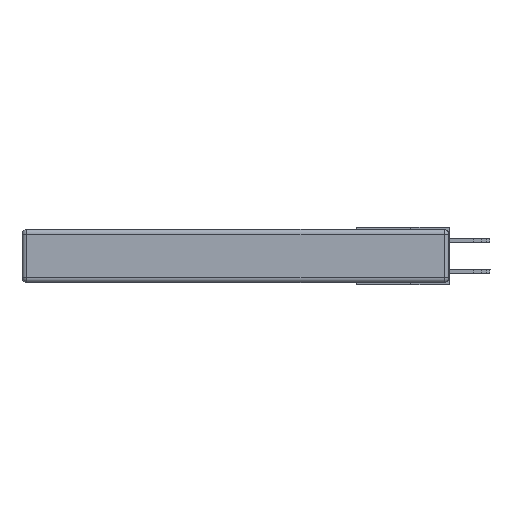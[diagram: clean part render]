
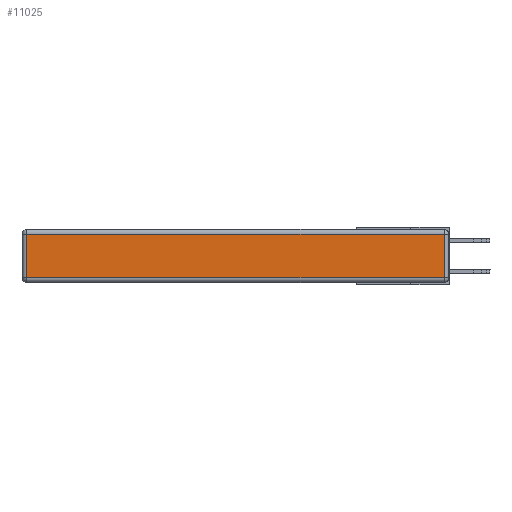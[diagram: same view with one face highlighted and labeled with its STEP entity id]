
A CAD part, left-side view. The second image highlights one B-rep face of the part: STEP entity #11025.
In plain terms, the highlighted planar face has unit normal (-1, 0, 0).
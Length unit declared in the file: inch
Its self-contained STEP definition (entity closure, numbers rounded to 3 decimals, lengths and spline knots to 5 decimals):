
#323 = DIRECTION ( 'NONE',  ( 0., -1., 0. ) ) ;
#461 = AXIS2_PLACEMENT_3D ( 'NONE', #13954, #5909, #7148 ) ;
#526 = VECTOR ( 'NONE', #9962, 39.37008 ) ;
#1801 = LINE ( 'NONE', #3574, #526 ) ;
#1982 = CARTESIAN_POINT ( 'NONE',  ( 0., 0.03, -0.313 ) ) ;
#2169 = DIRECTION ( 'NONE',  ( 0., 1., 0. ) ) ;
#2278 = VERTEX_POINT ( 'NONE', #8312 ) ;
#3091 = EDGE_CURVE ( 'NONE', #2278, #4308, #16827, .T. ) ;
#3574 = CARTESIAN_POINT ( 'NONE',  ( 0., 0.03, -0.343 ) ) ;
#4308 = VERTEX_POINT ( 'NONE', #16185 ) ;
#4618 = DIRECTION ( 'NONE',  ( 0., 0., -1. ) ) ;
#4994 = VECTOR ( 'NONE', #2169, 39.37008 ) ;
#5675 = CARTESIAN_POINT ( 'NONE',  ( 0., 0., -0.313 ) ) ;
#5909 = DIRECTION ( 'NONE',  ( -1., 0., 0. ) ) ;
#6187 = CARTESIAN_POINT ( 'NONE',  ( 0., 2.75, -0.03 ) ) ;
#6301 = CARTESIAN_POINT ( 'NONE',  ( 0., 0.03, -0.03 ) ) ;
#6712 = VECTOR ( 'NONE', #4618, 39.37008 ) ;
#7148 = DIRECTION ( 'NONE',  ( 0., 0., 1. ) ) ;
#7435 = CARTESIAN_POINT ( 'NONE',  ( 0., 2.72, -0.343 ) ) ;
#8312 = CARTESIAN_POINT ( 'NONE',  ( 0., 2.72, -0.03 ) ) ;
#9962 = DIRECTION ( 'NONE',  ( 0., 0., 1. ) ) ;
#11025 = ADVANCED_FACE ( 'NONE', ( #12907 ), #14008, .T. ) ;
#11042 = LINE ( 'NONE', #6187, #4994 ) ;
#11563 = ORIENTED_EDGE ( 'NONE', *, *, #17125, .T. ) ;
#11615 = ORIENTED_EDGE ( 'NONE', *, *, #3091, .T. ) ;
#12907 = FACE_OUTER_BOUND ( 'NONE', #13863, .T. ) ;
#13819 = VERTEX_POINT ( 'NONE', #1982 ) ;
#13863 = EDGE_LOOP ( 'NONE', ( #16670, #15102, #11563, #11615 ) ) ;
#13954 = CARTESIAN_POINT ( 'NONE',  ( 0., 0., -0.343 ) ) ;
#14008 = PLANE ( 'NONE',  #461 ) ;
#14283 = VERTEX_POINT ( 'NONE', #6301 ) ;
#15102 = ORIENTED_EDGE ( 'NONE', *, *, #17102, .T. ) ;
#15620 = EDGE_CURVE ( 'NONE', #4308, #13819, #17018, .T. ) ;
#16030 = VECTOR ( 'NONE', #323, 39.37008 ) ;
#16185 = CARTESIAN_POINT ( 'NONE',  ( 0., 2.72, -0.313 ) ) ;
#16670 = ORIENTED_EDGE ( 'NONE', *, *, #15620, .T. ) ;
#16827 = LINE ( 'NONE', #7435, #6712 ) ;
#17018 = LINE ( 'NONE', #5675, #16030 ) ;
#17102 = EDGE_CURVE ( 'NONE', #13819, #14283, #1801, .T. ) ;
#17125 = EDGE_CURVE ( 'NONE', #14283, #2278, #11042, .T. ) ;
